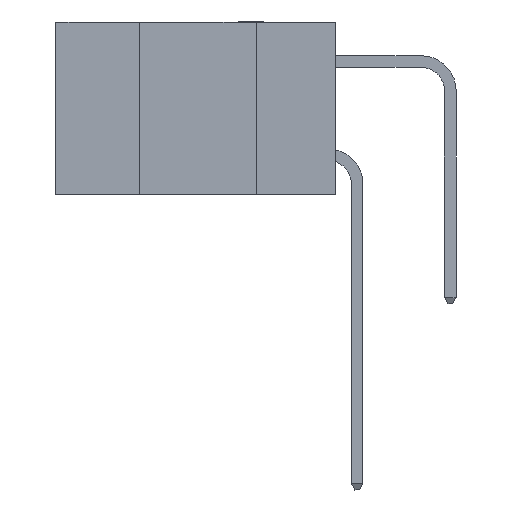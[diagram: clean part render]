
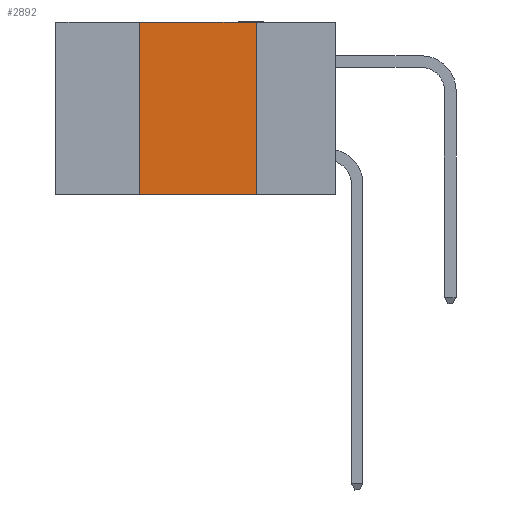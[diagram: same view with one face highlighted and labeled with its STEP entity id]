
A CAD part, left-side view. The second image highlights one B-rep face of the part: STEP entity #2892.
In plain terms, the highlighted planar face has unit normal (-1, 0, 0).
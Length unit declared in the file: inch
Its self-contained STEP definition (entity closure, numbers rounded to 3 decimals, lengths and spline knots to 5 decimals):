
#39 = EDGE_LOOP ( 'NONE', ( #36664, #30294, #20897, #3670 ) ) ;
#2892 = ADVANCED_FACE ( 'NONE', ( #10238 ), #19680, .F. ) ;
#3266 = CARTESIAN_POINT ( 'NONE',  ( 0., 0.17, 0. ) ) ;
#3670 = ORIENTED_EDGE ( 'NONE', *, *, #15817, .T. ) ;
#3881 = DIRECTION ( 'NONE',  ( 0., 0., -1. ) ) ;
#7827 = DIRECTION ( 'NONE',  ( 0., -1., 0. ) ) ;
#7903 = VECTOR ( 'NONE', #10050, 39.37008 ) ;
#8205 = CARTESIAN_POINT ( 'NONE',  ( 0., 0.6, -0.37 ) ) ;
#9050 = DIRECTION ( 'NONE',  ( 0., 0., -1. ) ) ;
#10050 = DIRECTION ( 'NONE',  ( 0., -1., 0. ) ) ;
#10238 = FACE_OUTER_BOUND ( 'NONE', #39, .T. ) ;
#11644 = CARTESIAN_POINT ( 'NONE',  ( 0., 0.42, -0.37 ) ) ;
#11992 = CARTESIAN_POINT ( 'NONE',  ( 0., 0.42, 0. ) ) ;
#13838 = LINE ( 'NONE', #3266, #34132 ) ;
#14578 = LINE ( 'NONE', #8205, #7903 ) ;
#15817 = EDGE_CURVE ( 'NONE', #28442, #19000, #14578, .T. ) ;
#15893 = DIRECTION ( 'NONE',  ( 0., 0., 1. ) ) ;
#16697 = AXIS2_PLACEMENT_3D ( 'NONE', #31905, #26722, #3881 ) ;
#18658 = VERTEX_POINT ( 'NONE', #11992 ) ;
#19000 = VERTEX_POINT ( 'NONE', #30346 ) ;
#19680 = PLANE ( 'NONE',  #16697 ) ;
#20069 = EDGE_CURVE ( 'NONE', #28648, #19000, #13838, .T. ) ;
#20897 = ORIENTED_EDGE ( 'NONE', *, *, #34282, .F. ) ;
#23328 = CARTESIAN_POINT ( 'NONE',  ( 0., 0.17, 0. ) ) ;
#24245 = LINE ( 'NONE', #27205, #25535 ) ;
#25535 = VECTOR ( 'NONE', #15893, 39.37008 ) ;
#26722 = DIRECTION ( 'NONE',  ( 1., 0., 0. ) ) ;
#27205 = CARTESIAN_POINT ( 'NONE',  ( 0., 0.42, 0. ) ) ;
#28442 = VERTEX_POINT ( 'NONE', #11644 ) ;
#28648 = VERTEX_POINT ( 'NONE', #23328 ) ;
#29149 = LINE ( 'NONE', #36256, #36407 ) ;
#30294 = ORIENTED_EDGE ( 'NONE', *, *, #33837, .F. ) ;
#30346 = CARTESIAN_POINT ( 'NONE',  ( 0., 0.17, -0.37 ) ) ;
#31905 = CARTESIAN_POINT ( 'NONE',  ( 0., 0.6, 0. ) ) ;
#33837 = EDGE_CURVE ( 'NONE', #18658, #28648, #29149, .T. ) ;
#34132 = VECTOR ( 'NONE', #9050, 39.37008 ) ;
#34282 = EDGE_CURVE ( 'NONE', #28442, #18658, #24245, .T. ) ;
#36256 = CARTESIAN_POINT ( 'NONE',  ( 0., 0.6, 0. ) ) ;
#36407 = VECTOR ( 'NONE', #7827, 39.37008 ) ;
#36664 = ORIENTED_EDGE ( 'NONE', *, *, #20069, .F. ) ;
